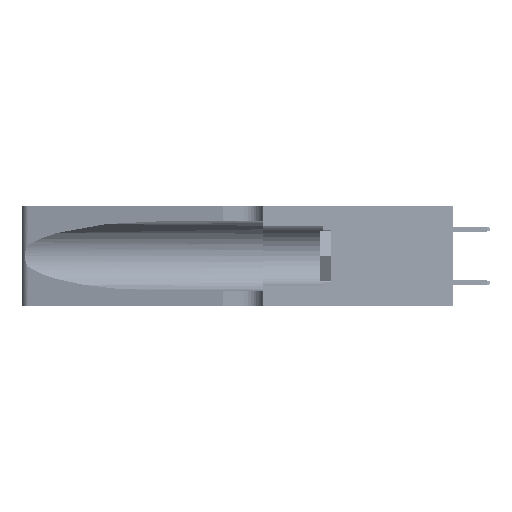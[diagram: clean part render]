
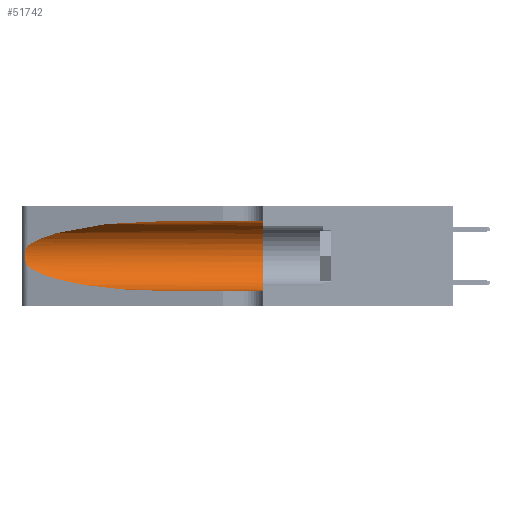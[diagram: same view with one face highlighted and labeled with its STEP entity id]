
A CAD part, left-side view. The second image highlights one B-rep face of the part: STEP entity #51742.
In plain terms, the highlighted cylindrical face has radius 3.308 mm (diameter 6.617 mm), a partial arc.
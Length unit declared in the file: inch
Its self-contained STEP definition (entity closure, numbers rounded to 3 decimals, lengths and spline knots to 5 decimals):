
#1309 = CARTESIAN_POINT ( 'NONE',  ( 0.1305, 1.61858, 0.185 ) ) ;
#4641 = CARTESIAN_POINT ( 'NONE',  ( 0.1305, 1.61858, 0.31525 ) ) ;
#4961 = CARTESIAN_POINT ( 'NONE',  ( 0.18966, 0.96281, 0.05475 ) ) ;
#5159 = EDGE_CURVE ( 'NONE', #9632, #16466, #36594, .T. ) ;
#5212 = EDGE_CURVE ( 'NONE', #48802, #16466, #27819, .T. ) ;
#5467 = ORIENTED_EDGE ( 'NONE', *, *, #5159, .T. ) ;
#6059 = CARTESIAN_POINT ( 'NONE',  ( 0.1305, 0.72297, 0.31525 ) ) ;
#6309 = CARTESIAN_POINT ( 'NONE',  ( 0.26075, 1.23896, 0.178 ) ) ;
#6389 =( BOUNDED_CURVE ( )  B_SPLINE_CURVE ( 3, ( #13100, #51007, #4961, #46411 ),
 .UNSPECIFIED., .F., .F. ) 
 B_SPLINE_CURVE_WITH_KNOTS ( ( 4, 4 ),
 ( 3.44316, 4.71239 ),
 .UNSPECIFIED. ) 
 CURVE ( )  GEOMETRIC_REPRESENTATION_ITEM ( )  RATIONAL_B_SPLINE_CURVE ( ( 1., 0.87, 0.87, 1. ) ) 
 REPRESENTATION_ITEM ( '' )  );
#6463 = VERTEX_POINT ( 'NONE', #28457 ) ;
#7836 = DIRECTION ( 'NONE',  ( 0., -1., 0. ) ) ;
#9301 = ORIENTED_EDGE ( 'NONE', *, *, #37914, .T. ) ;
#9632 = VERTEX_POINT ( 'NONE', #40070 ) ;
#10694 = CARTESIAN_POINT ( 'NONE',  ( 0.25487, 1.22718, 0.14631 ) ) ;
#11223 = CARTESIAN_POINT ( 'NONE',  ( 0.25639, 1.23186, 0.15144 ) ) ;
#13100 = CARTESIAN_POINT ( 'NONE',  ( 0.25487, 1.22718, 0.14631 ) ) ;
#13283 = FACE_OUTER_BOUND ( 'NONE', #39308, .T. ) ;
#15270 = CARTESIAN_POINT ( 'NONE',  ( 0.26075, 1.23896, 0.19203 ) ) ;
#15938 = EDGE_CURVE ( 'NONE', #48666, #24795, #49348, .T. ) ;
#16466 = VERTEX_POINT ( 'NONE', #48043 ) ;
#16830 = DIRECTION ( 'NONE',  ( 0., -1., 0. ) ) ;
#17327 = CYLINDRICAL_SURFACE ( 'NONE', #19524, 0.13025 ) ;
#18297 = CARTESIAN_POINT ( 'NONE',  ( 0.18966, 0.96281, 0.31525 ) ) ;
#18790 = CARTESIAN_POINT ( 'NONE',  ( 0.25555, 1.22993, 0.14849 ) ) ;
#19339 = CARTESIAN_POINT ( 'NONE',  ( 0.26018, 1.23835, 0.19895 ) ) ;
#19524 = AXIS2_PLACEMENT_3D ( 'NONE', #1309, #30873, #22426 ) ;
#21243 = CARTESIAN_POINT ( 'NONE',  ( 0.25487, 1.22718, 0.22369 ) ) ;
#21569 = ORIENTED_EDGE ( 'NONE', *, *, #34093, .T. ) ;
#21624 = DIRECTION ( 'NONE',  ( 0., 1., 0. ) ) ;
#21701 = B_SPLINE_CURVE_WITH_KNOTS ( 'NONE', 3,
 ( #32111, #52408, #47516, #43152, #27473, #19339, #15270, #6309, #26913, #48333, #40200, #11223, #18790, #10694 ),
 .UNSPECIFIED., .F., .F.,
 ( 4, 2, 2, 2, 2, 2, 4 ),
 ( 0., 0.00027, 0.00053, 0.00107, 0.0016, 0.00187, 0.00214 ),
 .UNSPECIFIED. ) ;
#22426 = DIRECTION ( 'NONE',  ( 0., 0., -1. ) ) ;
#22899 = CARTESIAN_POINT ( 'NONE',  ( 0.2373, 1.15595, 0.28018 ) ) ;
#23874 = EDGE_CURVE ( 'NONE', #48666, #48802, #37473, .T. ) ;
#24795 = VERTEX_POINT ( 'NONE', #21243 ) ;
#26913 = CARTESIAN_POINT ( 'NONE',  ( 0.26017, 1.23833, 0.17102 ) ) ;
#27473 = CARTESIAN_POINT ( 'NONE',  ( 0.25854, 1.2359, 0.20912 ) ) ;
#27768 = CARTESIAN_POINT ( 'NONE',  ( 0.1305, 0.35, 0.31525 ) ) ;
#27819 = CIRCLE ( 'NONE', #48596, 0.13025 ) ;
#28457 = CARTESIAN_POINT ( 'NONE',  ( 0.25487, 1.22718, 0.14631 ) ) ;
#29519 = DIRECTION ( 'NONE',  ( 0., 0., 1. ) ) ;
#30873 = DIRECTION ( 'NONE',  ( 0., -1., 0. ) ) ;
#32111 = CARTESIAN_POINT ( 'NONE',  ( 0.25487, 1.22718, 0.22369 ) ) ;
#34093 = EDGE_CURVE ( 'NONE', #24795, #6463, #21701, .T. ) ;
#34378 = CARTESIAN_POINT ( 'NONE',  ( 0.1305, 0.72297, 0.31525 ) ) ;
#36594 = LINE ( 'NONE', #53106, #44237 ) ;
#37473 = LINE ( 'NONE', #4641, #42897 ) ;
#37914 = EDGE_CURVE ( 'NONE', #6463, #9632, #6389, .T. ) ;
#38665 = ORIENTED_EDGE ( 'NONE', *, *, #23874, .F. ) ;
#39308 = EDGE_LOOP ( 'NONE', ( #48623, #21569, #9301, #5467, #51842, #38665 ) ) ;
#40070 = CARTESIAN_POINT ( 'NONE',  ( 0.1305, 0.72297, 0.05475 ) ) ;
#40200 = CARTESIAN_POINT ( 'NONE',  ( 0.25789, 1.23486, 0.15765 ) ) ;
#42231 = CARTESIAN_POINT ( 'NONE',  ( 0.1305, 0.35, 0.185 ) ) ;
#42897 = VECTOR ( 'NONE', #16830, 39.37008 ) ;
#43152 = CARTESIAN_POINT ( 'NONE',  ( 0.25787, 1.23484, 0.2124 ) ) ;
#44237 = VECTOR ( 'NONE', #7836, 39.37008 ) ;
#46411 = CARTESIAN_POINT ( 'NONE',  ( 0.1305, 0.72297, 0.05475 ) ) ;
#47516 = CARTESIAN_POINT ( 'NONE',  ( 0.25639, 1.23184, 0.21858 ) ) ;
#48043 = CARTESIAN_POINT ( 'NONE',  ( 0.1305, 0.35, 0.05475 ) ) ;
#48333 = CARTESIAN_POINT ( 'NONE',  ( 0.25856, 1.23593, 0.16098 ) ) ;
#48596 = AXIS2_PLACEMENT_3D ( 'NONE', #42231, #21624, #29519 ) ;
#48623 = ORIENTED_EDGE ( 'NONE', *, *, #15938, .T. ) ;
#48666 = VERTEX_POINT ( 'NONE', #6059 ) ;
#48802 = VERTEX_POINT ( 'NONE', #27768 ) ;
#49348 =( BOUNDED_CURVE ( )  B_SPLINE_CURVE ( 3, ( #34378, #18297, #22899, #50864 ),
 .UNSPECIFIED., .F., .T. ) 
 B_SPLINE_CURVE_WITH_KNOTS ( ( 4, 4 ),
 ( 1.5708, 2.84003 ),
 .UNSPECIFIED. ) 
 CURVE ( )  GEOMETRIC_REPRESENTATION_ITEM ( )  RATIONAL_B_SPLINE_CURVE ( ( 1., 0.87, 0.87, 1. ) ) 
 REPRESENTATION_ITEM ( '' )  );
#50864 = CARTESIAN_POINT ( 'NONE',  ( 0.25487, 1.22718, 0.22369 ) ) ;
#51007 = CARTESIAN_POINT ( 'NONE',  ( 0.2373, 1.15595, 0.08982 ) ) ;
#51742 = ADVANCED_FACE ( 'NONE', ( #13283 ), #17327, .F. ) ;
#51842 = ORIENTED_EDGE ( 'NONE', *, *, #5212, .F. ) ;
#52408 = CARTESIAN_POINT ( 'NONE',  ( 0.25555, 1.22994, 0.2215 ) ) ;
#53106 = CARTESIAN_POINT ( 'NONE',  ( 0.1305, 1.61858, 0.05475 ) ) ;
